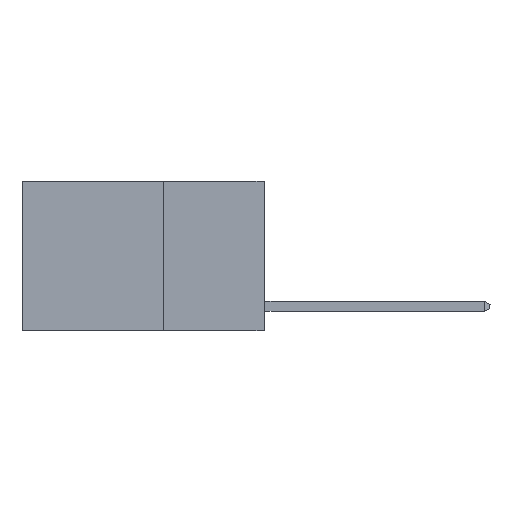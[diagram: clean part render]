
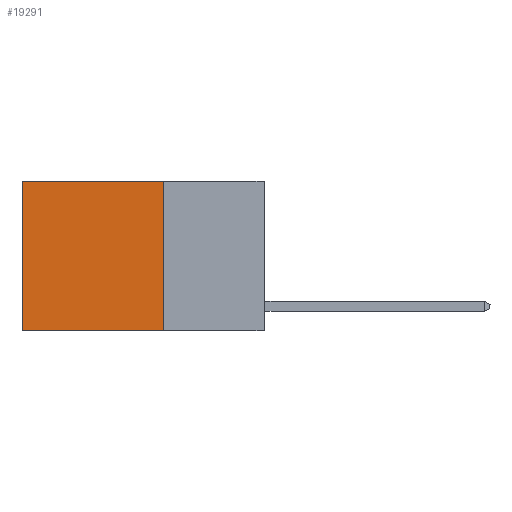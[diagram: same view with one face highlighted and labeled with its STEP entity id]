
A CAD part, left-side view. The second image highlights one B-rep face of the part: STEP entity #19291.
In plain terms, the highlighted planar face has unit normal (-1, 0, 0).
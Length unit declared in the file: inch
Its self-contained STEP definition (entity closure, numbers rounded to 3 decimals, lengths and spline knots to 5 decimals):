
#617 = VECTOR ( 'NONE', #17310, 39.37008 ) ;
#747 = DIRECTION ( 'NONE',  ( 0., 1., 0. ) ) ;
#1281 = CARTESIAN_POINT ( 'NONE',  ( 0.2625, 0.25, 0. ) ) ;
#1423 = DIRECTION ( 'NONE',  ( 1., 0., 0. ) ) ;
#1964 = CARTESIAN_POINT ( 'NONE',  ( 0.2625, 0.25, 0. ) ) ;
#2315 = ORIENTED_EDGE ( 'NONE', *, *, #8465, .F. ) ;
#2556 = CARTESIAN_POINT ( 'NONE',  ( 0.2625, 0.25, -0.37 ) ) ;
#4511 = VECTOR ( 'NONE', #18290, 39.37008 ) ;
#4517 = VERTEX_POINT ( 'NONE', #26760 ) ;
#5222 = LINE ( 'NONE', #2556, #4511 ) ;
#5888 = LINE ( 'NONE', #19105, #14963 ) ;
#7380 = CARTESIAN_POINT ( 'NONE',  ( 0.2625, 0.25, 0. ) ) ;
#7646 = FACE_OUTER_BOUND ( 'NONE', #17546, .T. ) ;
#8092 = ORIENTED_EDGE ( 'NONE', *, *, #11577, .T. ) ;
#8465 = EDGE_CURVE ( 'NONE', #14591, #11486, #5888, .T. ) ;
#11486 = VERTEX_POINT ( 'NONE', #25291 ) ;
#11577 = EDGE_CURVE ( 'NONE', #4517, #16672, #22663, .T. ) ;
#12634 = CARTESIAN_POINT ( 'NONE',  ( 0.2625, 0.6, -0.37 ) ) ;
#13248 = ORIENTED_EDGE ( 'NONE', *, *, #21433, .F. ) ;
#14591 = VERTEX_POINT ( 'NONE', #1964 ) ;
#14767 = DIRECTION ( 'NONE',  ( 0., 0., -1. ) ) ;
#14963 = VECTOR ( 'NONE', #14767, 39.37008 ) ;
#16218 = DIRECTION ( 'NONE',  ( 0., 0., -1. ) ) ;
#16672 = VERTEX_POINT ( 'NONE', #12634 ) ;
#17310 = DIRECTION ( 'NONE',  ( 0., 0., -1. ) ) ;
#17546 = EDGE_LOOP ( 'NONE', ( #8092, #13248, #2315, #18090 ) ) ;
#18090 = ORIENTED_EDGE ( 'NONE', *, *, #21007, .T. ) ;
#18290 = DIRECTION ( 'NONE',  ( 0., 1., 0. ) ) ;
#19105 = CARTESIAN_POINT ( 'NONE',  ( 0.2625, 0.25, 0. ) ) ;
#19291 = ADVANCED_FACE ( 'NONE', ( #7646 ), #20690, .F. ) ;
#20690 = PLANE ( 'NONE',  #27294 ) ;
#21007 = EDGE_CURVE ( 'NONE', #14591, #4517, #26320, .T. ) ;
#21433 = EDGE_CURVE ( 'NONE', #11486, #16672, #5222, .T. ) ;
#21801 = CARTESIAN_POINT ( 'NONE',  ( 0.2625, 0.6, 0. ) ) ;
#22663 = LINE ( 'NONE', #21801, #617 ) ;
#23329 = VECTOR ( 'NONE', #747, 39.37008 ) ;
#25291 = CARTESIAN_POINT ( 'NONE',  ( 0.2625, 0.25, -0.37 ) ) ;
#26320 = LINE ( 'NONE', #7380, #23329 ) ;
#26760 = CARTESIAN_POINT ( 'NONE',  ( 0.2625, 0.6, 0. ) ) ;
#27294 = AXIS2_PLACEMENT_3D ( 'NONE', #1281, #1423, #16218 ) ;
